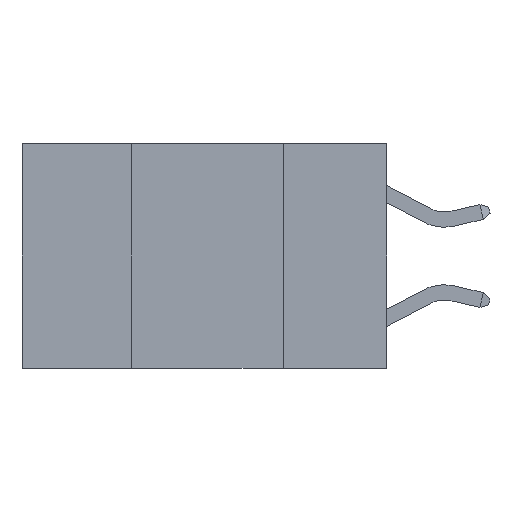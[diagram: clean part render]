
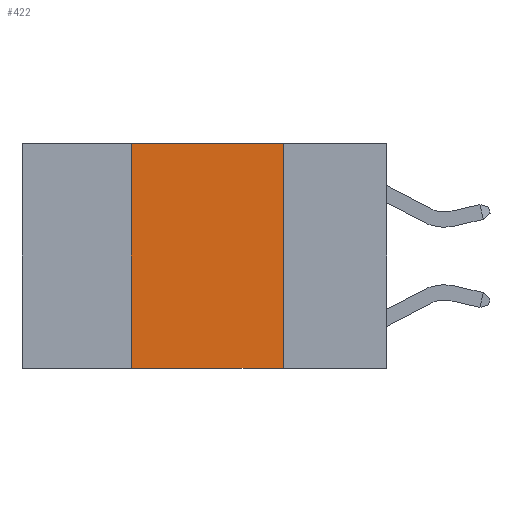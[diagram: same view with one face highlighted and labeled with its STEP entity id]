
A CAD part, left-side view. The second image highlights one B-rep face of the part: STEP entity #422.
In plain terms, the highlighted planar face has unit normal (-1, 0, 0).
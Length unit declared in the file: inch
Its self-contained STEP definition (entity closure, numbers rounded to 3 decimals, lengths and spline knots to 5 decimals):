
#188 = ORIENTED_EDGE ( 'NONE', *, *, #10869, .F. ) ;
#422 = ADVANCED_FACE ( 'NONE', ( #2733 ), #15714, .F. ) ;
#447 = CARTESIAN_POINT ( 'NONE',  ( 0., 0.17, 0. ) ) ;
#624 = CARTESIAN_POINT ( 'NONE',  ( 0., 0.6, -0.37 ) ) ;
#1398 = LINE ( 'NONE', #9798, #4558 ) ;
#2083 = VERTEX_POINT ( 'NONE', #12285 ) ;
#2194 = EDGE_CURVE ( 'NONE', #8073, #6503, #1398, .T. ) ;
#2733 = FACE_OUTER_BOUND ( 'NONE', #15171, .T. ) ;
#3090 = LINE ( 'NONE', #13555, #13496 ) ;
#3176 = VECTOR ( 'NONE', #15032, 39.37008 ) ;
#4558 = VECTOR ( 'NONE', #5812, 39.37008 ) ;
#5812 = DIRECTION ( 'NONE',  ( 0., 0., -1. ) ) ;
#6123 = EDGE_CURVE ( 'NONE', #17406, #6503, #11638, .T. ) ;
#6205 = CARTESIAN_POINT ( 'NONE',  ( 0., 0.6, 0. ) ) ;
#6503 = VERTEX_POINT ( 'NONE', #10868 ) ;
#6525 = ORIENTED_EDGE ( 'NONE', *, *, #2194, .F. ) ;
#7281 = AXIS2_PLACEMENT_3D ( 'NONE', #6205, #7581, #17089 ) ;
#7388 = ORIENTED_EDGE ( 'NONE', *, *, #14964, .F. ) ;
#7581 = DIRECTION ( 'NONE',  ( 1., 0., 0. ) ) ;
#8073 = VERTEX_POINT ( 'NONE', #447 ) ;
#9798 = CARTESIAN_POINT ( 'NONE',  ( 0., 0.17, 0. ) ) ;
#10868 = CARTESIAN_POINT ( 'NONE',  ( 0., 0.17, -0.37 ) ) ;
#10869 = EDGE_CURVE ( 'NONE', #2083, #8073, #3090, .T. ) ;
#11217 = VECTOR ( 'NONE', #11465, 39.37008 ) ;
#11465 = DIRECTION ( 'NONE',  ( 0., -1., 0. ) ) ;
#11638 = LINE ( 'NONE', #624, #11217 ) ;
#12285 = CARTESIAN_POINT ( 'NONE',  ( 0., 0.42, 0. ) ) ;
#13422 = CARTESIAN_POINT ( 'NONE',  ( 0., 0.42, -0.37 ) ) ;
#13496 = VECTOR ( 'NONE', #14905, 39.37008 ) ;
#13555 = CARTESIAN_POINT ( 'NONE',  ( 0., 0.6, 0. ) ) ;
#14027 = LINE ( 'NONE', #16395, #3176 ) ;
#14616 = ORIENTED_EDGE ( 'NONE', *, *, #6123, .T. ) ;
#14905 = DIRECTION ( 'NONE',  ( 0., -1., 0. ) ) ;
#14964 = EDGE_CURVE ( 'NONE', #17406, #2083, #14027, .T. ) ;
#15032 = DIRECTION ( 'NONE',  ( 0., 0., 1. ) ) ;
#15171 = EDGE_LOOP ( 'NONE', ( #6525, #188, #7388, #14616 ) ) ;
#15714 = PLANE ( 'NONE',  #7281 ) ;
#16395 = CARTESIAN_POINT ( 'NONE',  ( 0., 0.42, 0. ) ) ;
#17089 = DIRECTION ( 'NONE',  ( 0., 0., -1. ) ) ;
#17406 = VERTEX_POINT ( 'NONE', #13422 ) ;
